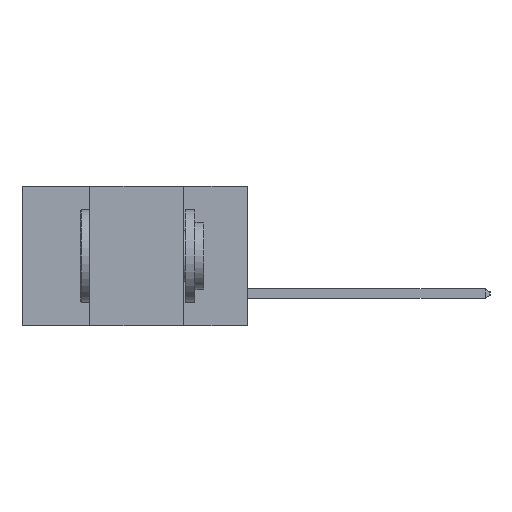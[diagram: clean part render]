
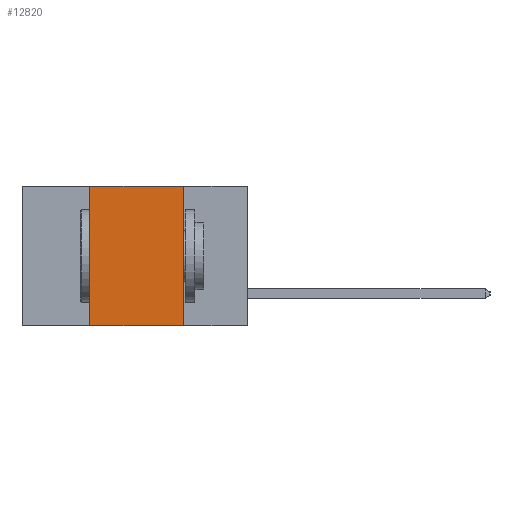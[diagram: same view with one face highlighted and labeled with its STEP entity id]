
A CAD part, left-side view. The second image highlights one B-rep face of the part: STEP entity #12820.
In plain terms, the highlighted planar face has unit normal (-1, 0, 0).
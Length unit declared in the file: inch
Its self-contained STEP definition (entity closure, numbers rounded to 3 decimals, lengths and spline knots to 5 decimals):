
#614 = VECTOR ( 'NONE', #11798, 39.37008 ) ;
#941 = VECTOR ( 'NONE', #10310, 39.37008 ) ;
#1418 = CARTESIAN_POINT ( 'NONE',  ( 0., 0.42, -0.37 ) ) ;
#1484 = EDGE_CURVE ( 'NONE', #17771, #20252, #15978, .T. ) ;
#3173 = CARTESIAN_POINT ( 'NONE',  ( 0., 0.42, 0. ) ) ;
#6503 = ORIENTED_EDGE ( 'NONE', *, *, #12434, .F. ) ;
#6559 = FACE_OUTER_BOUND ( 'NONE', #15047, .T. ) ;
#10241 = EDGE_CURVE ( 'NONE', #14545, #20252, #12882, .T. ) ;
#10310 = DIRECTION ( 'NONE',  ( 0., -1., 0. ) ) ;
#10358 = CARTESIAN_POINT ( 'NONE',  ( 0., 0.6, 0. ) ) ;
#11743 = AXIS2_PLACEMENT_3D ( 'NONE', #17531, #17819, #17334 ) ;
#11798 = DIRECTION ( 'NONE',  ( 0., 0., 1. ) ) ;
#12434 = EDGE_CURVE ( 'NONE', #16406, #14545, #19940, .T. ) ;
#12629 = ORIENTED_EDGE ( 'NONE', *, *, #10241, .F. ) ;
#12820 = ADVANCED_FACE ( 'NONE', ( #6559 ), #17271, .F. ) ;
#12837 = CARTESIAN_POINT ( 'NONE',  ( 0., 0.17, 0. ) ) ;
#12882 = LINE ( 'NONE', #20496, #17333 ) ;
#12993 = CARTESIAN_POINT ( 'NONE',  ( 0., 0.42, -0.37 ) ) ;
#13742 = LINE ( 'NONE', #12993, #614 ) ;
#14524 = EDGE_CURVE ( 'NONE', #17771, #16406, #13742, .T. ) ;
#14545 = VERTEX_POINT ( 'NONE', #12837 ) ;
#15047 = EDGE_LOOP ( 'NONE', ( #12629, #6503, #17254, #15575 ) ) ;
#15452 = VECTOR ( 'NONE', #18878, 39.37008 ) ;
#15575 = ORIENTED_EDGE ( 'NONE', *, *, #1484, .T. ) ;
#15978 = LINE ( 'NONE', #18413, #15452 ) ;
#16406 = VERTEX_POINT ( 'NONE', #3173 ) ;
#17254 = ORIENTED_EDGE ( 'NONE', *, *, #14524, .F. ) ;
#17271 = PLANE ( 'NONE',  #11743 ) ;
#17333 = VECTOR ( 'NONE', #20473, 39.37008 ) ;
#17334 = DIRECTION ( 'NONE',  ( 0., 0., -1. ) ) ;
#17531 = CARTESIAN_POINT ( 'NONE',  ( 0., 0.6, 0. ) ) ;
#17771 = VERTEX_POINT ( 'NONE', #1418 ) ;
#17819 = DIRECTION ( 'NONE',  ( 1., 0., 0. ) ) ;
#18413 = CARTESIAN_POINT ( 'NONE',  ( 0., 0.6, -0.37 ) ) ;
#18878 = DIRECTION ( 'NONE',  ( 0., -1., 0. ) ) ;
#19940 = LINE ( 'NONE', #10358, #941 ) ;
#20252 = VERTEX_POINT ( 'NONE', #20325 ) ;
#20325 = CARTESIAN_POINT ( 'NONE',  ( 0., 0.17, -0.37 ) ) ;
#20473 = DIRECTION ( 'NONE',  ( 0., 0., -1. ) ) ;
#20496 = CARTESIAN_POINT ( 'NONE',  ( 0., 0.17, -0.37 ) ) ;
